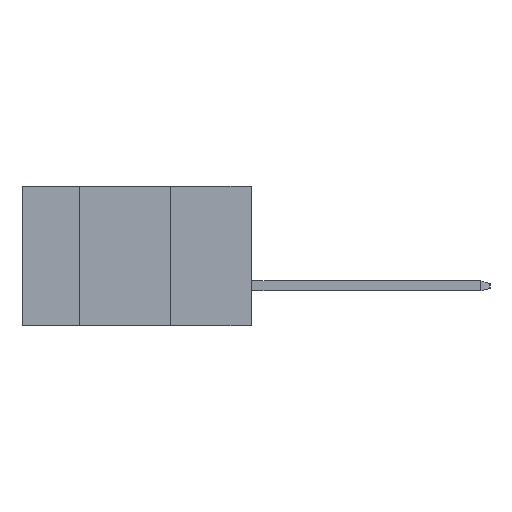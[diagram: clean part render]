
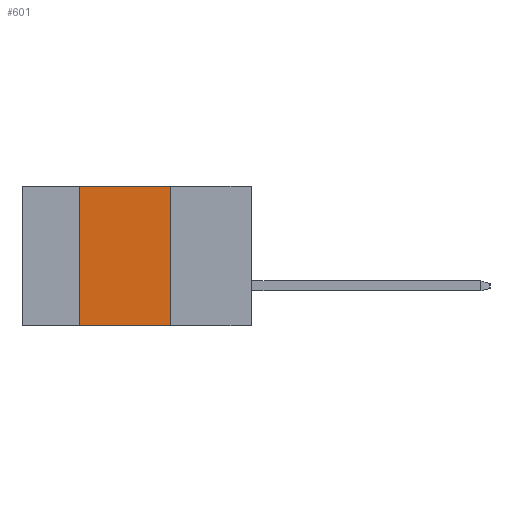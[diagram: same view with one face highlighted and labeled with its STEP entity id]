
A CAD part, left-side view. The second image highlights one B-rep face of the part: STEP entity #601.
In plain terms, the highlighted planar face has unit normal (-1, 0, 0).
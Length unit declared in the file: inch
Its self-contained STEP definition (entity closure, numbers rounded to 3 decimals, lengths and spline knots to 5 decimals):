
#10 = ORIENTED_EDGE ( 'NONE', *, *, #8819, .F. ) ;
#125 = EDGE_CURVE ( 'NONE', #11100, #427, #10233, .T. ) ;
#298 = VERTEX_POINT ( 'NONE', #7754 ) ;
#377 = LINE ( 'NONE', #10926, #3993 ) ;
#427 = VERTEX_POINT ( 'NONE', #5000 ) ;
#549 = EDGE_LOOP ( 'NONE', ( #12347, #2142, #10, #5648 ) ) ;
#601 = ADVANCED_FACE ( 'NONE', ( #7417 ), #8383, .F. ) ;
#1853 = VECTOR ( 'NONE', #7429, 39.37008 ) ;
#2142 = ORIENTED_EDGE ( 'NONE', *, *, #10347, .F. ) ;
#2254 = EDGE_CURVE ( 'NONE', #3632, #427, #10215, .T. ) ;
#2579 = DIRECTION ( 'NONE',  ( 1., 0., 0. ) ) ;
#3603 = DIRECTION ( 'NONE',  ( 0., 0., -1. ) ) ;
#3632 = VERTEX_POINT ( 'NONE', #5508 ) ;
#3666 = AXIS2_PLACEMENT_3D ( 'NONE', #11315, #2579, #3603 ) ;
#3902 = CARTESIAN_POINT ( 'NONE',  ( 0., 0.54, -0.437 ) ) ;
#3993 = VECTOR ( 'NONE', #10855, 39.37008 ) ;
#4825 = CARTESIAN_POINT ( 'NONE',  ( 0., 0.54, -0.437 ) ) ;
#5000 = CARTESIAN_POINT ( 'NONE',  ( 0., 0.254, -0.437 ) ) ;
#5508 = CARTESIAN_POINT ( 'NONE',  ( 0., 0.254, 0. ) ) ;
#5648 = ORIENTED_EDGE ( 'NONE', *, *, #125, .T. ) ;
#6891 = VECTOR ( 'NONE', #10275, 39.37008 ) ;
#7417 = FACE_OUTER_BOUND ( 'NONE', #549, .T. ) ;
#7429 = DIRECTION ( 'NONE',  ( 0., -1., 0. ) ) ;
#7754 = CARTESIAN_POINT ( 'NONE',  ( 0., 0.54, 0. ) ) ;
#8383 = PLANE ( 'NONE',  #3666 ) ;
#8819 = EDGE_CURVE ( 'NONE', #11100, #298, #9710, .T. ) ;
#9710 = LINE ( 'NONE', #3902, #10937 ) ;
#10215 = LINE ( 'NONE', #12397, #6891 ) ;
#10233 = LINE ( 'NONE', #12162, #1853 ) ;
#10275 = DIRECTION ( 'NONE',  ( 0., 0., -1. ) ) ;
#10347 = EDGE_CURVE ( 'NONE', #298, #3632, #377, .T. ) ;
#10855 = DIRECTION ( 'NONE',  ( 0., -1., 0. ) ) ;
#10926 = CARTESIAN_POINT ( 'NONE',  ( 0., 0.72, 0. ) ) ;
#10937 = VECTOR ( 'NONE', #11683, 39.37008 ) ;
#11100 = VERTEX_POINT ( 'NONE', #4825 ) ;
#11315 = CARTESIAN_POINT ( 'NONE',  ( 0., 0.72, 0. ) ) ;
#11683 = DIRECTION ( 'NONE',  ( 0., 0., 1. ) ) ;
#12162 = CARTESIAN_POINT ( 'NONE',  ( 0., 0.72, -0.437 ) ) ;
#12347 = ORIENTED_EDGE ( 'NONE', *, *, #2254, .F. ) ;
#12397 = CARTESIAN_POINT ( 'NONE',  ( 0., 0.254, -0.437 ) ) ;
